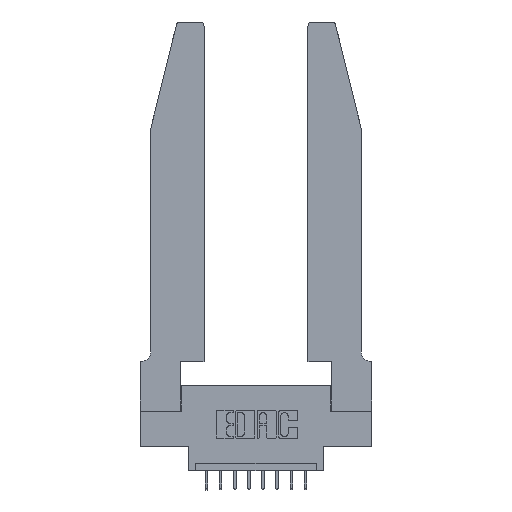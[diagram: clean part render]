
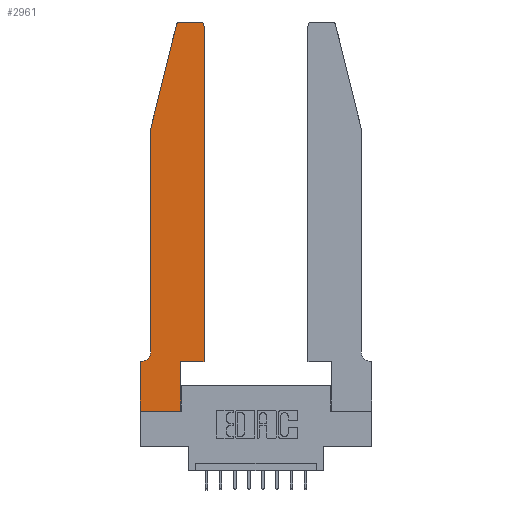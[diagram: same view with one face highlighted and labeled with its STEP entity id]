
A CAD part, top view. The second image highlights one B-rep face of the part: STEP entity #2961.
In plain terms, the highlighted planar face has unit normal (0, 0, 1).
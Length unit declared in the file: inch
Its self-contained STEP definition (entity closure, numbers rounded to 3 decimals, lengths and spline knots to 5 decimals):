
#116 = EDGE_CURVE ( 'NONE', #5776, #15455, #9686, .T. ) ;
#185 = DIRECTION ( 'NONE',  ( 0., 1., 0. ) ) ;
#697 = CARTESIAN_POINT ( 'NONE',  ( 0., 0., 0.37 ) ) ;
#855 = DIRECTION ( 'NONE',  ( 1., 0., 0. ) ) ;
#887 = VECTOR ( 'NONE', #3904, 39.37008 ) ;
#1096 = DIRECTION ( 'NONE',  ( -1., 0., 0. ) ) ;
#1345 = VECTOR ( 'NONE', #5711, 39.37008 ) ;
#1521 = LINE ( 'NONE', #8588, #887 ) ;
#1634 = VECTOR ( 'NONE', #12336, 39.37008 ) ;
#1656 = VECTOR ( 'NONE', #11247, 39.37008 ) ;
#1775 = CARTESIAN_POINT ( 'NONE',  ( 0.2865, 0.35, 0.37 ) ) ;
#2142 = LINE ( 'NONE', #15311, #1345 ) ;
#2153 = AXIS2_PLACEMENT_3D ( 'NONE', #6870, #5777, #12791 ) ;
#2532 = VERTEX_POINT ( 'NONE', #1775 ) ;
#2568 = PLANE ( 'NONE',  #6472 ) ;
#2575 = LINE ( 'NONE', #9648, #1634 ) ;
#2708 = VERTEX_POINT ( 'NONE', #10432 ) ;
#2842 = VECTOR ( 'NONE', #185, 39.37008 ) ;
#2961 = ADVANCED_FACE ( 'NONE', ( #6207 ), #2568, .T. ) ;
#3234 = EDGE_CURVE ( 'NONE', #4161, #2532, #2142, .T. ) ;
#3318 = LINE ( 'NONE', #10704, #7856 ) ;
#3413 = CARTESIAN_POINT ( 'NONE',  ( 0.4205, 2.72, 0.37 ) ) ;
#3501 = DIRECTION ( 'NONE',  ( 0., 0., 1. ) ) ;
#3504 = ORIENTED_EDGE ( 'NONE', *, *, #6648, .T. ) ;
#3731 = CIRCLE ( 'NONE', #5732, 0.03 ) ;
#3846 = CARTESIAN_POINT ( 'NONE',  ( 0.0755, 2., 0.37 ) ) ;
#3904 = DIRECTION ( 'NONE',  ( -1., 0., 0. ) ) ;
#4016 = VERTEX_POINT ( 'NONE', #12181 ) ;
#4109 = DIRECTION ( 'NONE',  ( 0., -1., 0. ) ) ;
#4161 = VERTEX_POINT ( 'NONE', #4376 ) ;
#4376 = CARTESIAN_POINT ( 'NONE',  ( 0.2865, 0., 0.37 ) ) ;
#4719 = CIRCLE ( 'NONE', #10727, 0.07 ) ;
#4827 = EDGE_CURVE ( 'NONE', #14307, #13596, #3318, .T. ) ;
#4991 = LINE ( 'NONE', #9833, #1656 ) ;
#5228 = VECTOR ( 'NONE', #4109, 39.37008 ) ;
#5277 = CARTESIAN_POINT ( 'NONE',  ( 0.0755, 0.42, 0.37 ) ) ;
#5680 = CARTESIAN_POINT ( 'NONE',  ( 0.284, 2.75, 0.37 ) ) ;
#5694 = ORIENTED_EDGE ( 'NONE', *, *, #15196, .T. ) ;
#5711 = DIRECTION ( 'NONE',  ( 0., 1., 0. ) ) ;
#5732 = AXIS2_PLACEMENT_3D ( 'NONE', #3413, #3501, #8265 ) ;
#5750 = LINE ( 'NONE', #697, #11582 ) ;
#5776 = VERTEX_POINT ( 'NONE', #11594 ) ;
#5777 = DIRECTION ( 'NONE',  ( 0., 0., 1. ) ) ;
#5946 = CARTESIAN_POINT ( 'NONE',  ( 0.4205, 2.75, 0.37 ) ) ;
#6001 = ORIENTED_EDGE ( 'NONE', *, *, #7574, .T. ) ;
#6182 = CARTESIAN_POINT ( 'NONE',  ( 0.4505, 0.35, 0.37 ) ) ;
#6207 = FACE_OUTER_BOUND ( 'NONE', #7378, .T. ) ;
#6403 = CARTESIAN_POINT ( 'NONE',  ( 0., 0., 0.37 ) ) ;
#6472 = AXIS2_PLACEMENT_3D ( 'NONE', #8743, #12401, #7359 ) ;
#6648 = EDGE_CURVE ( 'NONE', #13330, #15381, #1521, .T. ) ;
#6870 = CARTESIAN_POINT ( 'NONE',  ( 0.284, 2.72, 0.37 ) ) ;
#7093 = ORIENTED_EDGE ( 'NONE', *, *, #8824, .T. ) ;
#7187 = CARTESIAN_POINT ( 'NONE',  ( 0.0055, 0.35, 0.37 ) ) ;
#7215 = ORIENTED_EDGE ( 'NONE', *, *, #9511, .T. ) ;
#7252 = VERTEX_POINT ( 'NONE', #8205 ) ;
#7296 = LINE ( 'NONE', #3846, #15236 ) ;
#7359 = DIRECTION ( 'NONE',  ( 1., 0., 0. ) ) ;
#7378 = EDGE_LOOP ( 'NONE', ( #8956, #13451, #6001, #7619, #7093, #3504, #7215, #5694, #8338, #11014, #10979, #15434 ) ) ;
#7521 = EDGE_CURVE ( 'NONE', #7252, #8654, #7296, .T. ) ;
#7574 = EDGE_CURVE ( 'NONE', #4016, #7252, #2575, .T. ) ;
#7619 = ORIENTED_EDGE ( 'NONE', *, *, #7521, .T. ) ;
#7645 = EDGE_CURVE ( 'NONE', #13596, #4016, #13976, .T. ) ;
#7856 = VECTOR ( 'NONE', #12057, 39.37008 ) ;
#8205 = CARTESIAN_POINT ( 'NONE',  ( 0.0755, 2., 0.37 ) ) ;
#8265 = DIRECTION ( 'NONE',  ( 1., 0., 0. ) ) ;
#8309 = CARTESIAN_POINT ( 'NONE',  ( 0., 0.35, 0.37 ) ) ;
#8338 = ORIENTED_EDGE ( 'NONE', *, *, #3234, .T. ) ;
#8588 = CARTESIAN_POINT ( 'NONE',  ( 0.0755, 0.35, 0.37 ) ) ;
#8622 = EDGE_CURVE ( 'NONE', #2532, #5776, #4991, .T. ) ;
#8654 = VERTEX_POINT ( 'NONE', #5277 ) ;
#8743 = CARTESIAN_POINT ( 'NONE',  ( 0., 0.35, 0.37 ) ) ;
#8824 = EDGE_CURVE ( 'NONE', #8654, #13330, #4719, .T. ) ;
#8956 = ORIENTED_EDGE ( 'NONE', *, *, #4827, .T. ) ;
#9511 = EDGE_CURVE ( 'NONE', #15381, #2708, #12455, .T. ) ;
#9648 = CARTESIAN_POINT ( 'NONE',  ( 0.0755, 2., 0.37 ) ) ;
#9686 = LINE ( 'NONE', #6182, #2842 ) ;
#9833 = CARTESIAN_POINT ( 'NONE',  ( 0.4505, 0.35, 0.37 ) ) ;
#9877 = DIRECTION ( 'NONE',  ( 0., -1., 0. ) ) ;
#10432 = CARTESIAN_POINT ( 'NONE',  ( 0., 0., 0.37 ) ) ;
#10704 = CARTESIAN_POINT ( 'NONE',  ( 0.2605, 2.75, 0.37 ) ) ;
#10727 = AXIS2_PLACEMENT_3D ( 'NONE', #10850, #11882, #1096 ) ;
#10850 = CARTESIAN_POINT ( 'NONE',  ( 0.0055, 0.42, 0.37 ) ) ;
#10979 = ORIENTED_EDGE ( 'NONE', *, *, #116, .T. ) ;
#11014 = ORIENTED_EDGE ( 'NONE', *, *, #8622, .T. ) ;
#11071 = EDGE_CURVE ( 'NONE', #15455, #14307, #3731, .T. ) ;
#11247 = DIRECTION ( 'NONE',  ( 1., 0., 0. ) ) ;
#11582 = VECTOR ( 'NONE', #855, 39.37008 ) ;
#11594 = CARTESIAN_POINT ( 'NONE',  ( 0.4505, 0.35, 0.37 ) ) ;
#11882 = DIRECTION ( 'NONE',  ( 0., 0., -1. ) ) ;
#12057 = DIRECTION ( 'NONE',  ( -1., 0., 0. ) ) ;
#12181 = CARTESIAN_POINT ( 'NONE',  ( 0.25487, 2.72718, 0.37 ) ) ;
#12268 = CARTESIAN_POINT ( 'NONE',  ( 0.4505, 2.72, 0.37 ) ) ;
#12336 = DIRECTION ( 'NONE',  ( -0.239, -0.971, 0. ) ) ;
#12401 = DIRECTION ( 'NONE',  ( 0., 0., 1. ) ) ;
#12455 = LINE ( 'NONE', #6403, #5228 ) ;
#12791 = DIRECTION ( 'NONE',  ( 1., 0., 0. ) ) ;
#13330 = VERTEX_POINT ( 'NONE', #7187 ) ;
#13451 = ORIENTED_EDGE ( 'NONE', *, *, #7645, .T. ) ;
#13596 = VERTEX_POINT ( 'NONE', #5680 ) ;
#13976 = CIRCLE ( 'NONE', #2153, 0.03 ) ;
#14307 = VERTEX_POINT ( 'NONE', #5946 ) ;
#15196 = EDGE_CURVE ( 'NONE', #2708, #4161, #5750, .T. ) ;
#15236 = VECTOR ( 'NONE', #9877, 39.37008 ) ;
#15311 = CARTESIAN_POINT ( 'NONE',  ( 0.2865, 0.35, 0.37 ) ) ;
#15381 = VERTEX_POINT ( 'NONE', #8309 ) ;
#15434 = ORIENTED_EDGE ( 'NONE', *, *, #11071, .T. ) ;
#15455 = VERTEX_POINT ( 'NONE', #12268 ) ;
